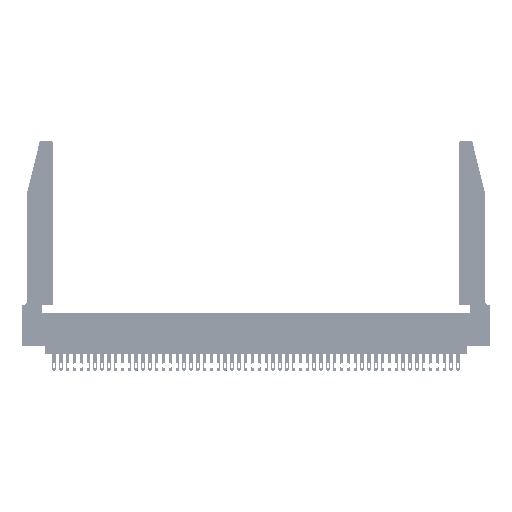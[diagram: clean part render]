
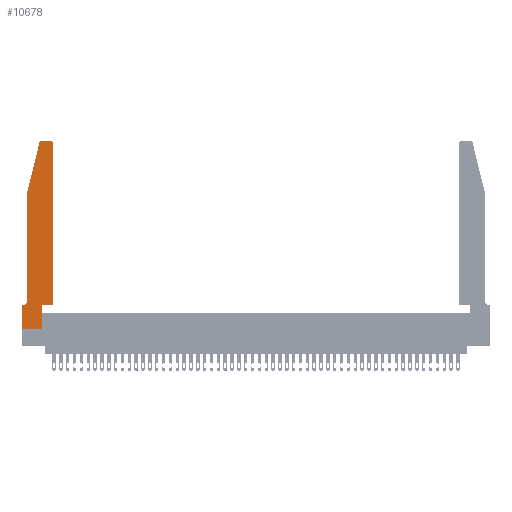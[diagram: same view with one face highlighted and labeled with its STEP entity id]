
A CAD part, top view. The second image highlights one B-rep face of the part: STEP entity #10678.
In plain terms, the highlighted planar face has unit normal (0, 0, 1).
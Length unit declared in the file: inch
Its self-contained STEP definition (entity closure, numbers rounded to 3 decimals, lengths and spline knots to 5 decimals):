
#376 = CARTESIAN_POINT ( 'NONE',  ( 0., 0., 0.37 ) ) ;
#526 = EDGE_CURVE ( 'NONE', #38682, #22160, #24939, .T. ) ;
#804 = EDGE_CURVE ( 'NONE', #26016, #16310, #4045, .T. ) ;
#1109 = CARTESIAN_POINT ( 'NONE',  ( 0.2865, 0.35, 0.37 ) ) ;
#1453 = DIRECTION ( 'NONE',  ( 0., 1., 0. ) ) ;
#1517 = CARTESIAN_POINT ( 'NONE',  ( 0.0055, 0.35, 0.37 ) ) ;
#1753 = CARTESIAN_POINT ( 'NONE',  ( 0.284, 2.72, 0.37 ) ) ;
#2973 = CARTESIAN_POINT ( 'NONE',  ( 0.284, 2.75, 0.37 ) ) ;
#3217 = DIRECTION ( 'NONE',  ( 0., -1., 0. ) ) ;
#3807 = CARTESIAN_POINT ( 'NONE',  ( 0.4505, 2.72, 0.37 ) ) ;
#4045 = LINE ( 'NONE', #29540, #39328 ) ;
#4245 = ORIENTED_EDGE ( 'NONE', *, *, #41643, .T. ) ;
#4680 = AXIS2_PLACEMENT_3D ( 'NONE', #41385, #18926, #25954 ) ;
#5429 = DIRECTION ( 'NONE',  ( 1., 0., 0. ) ) ;
#6351 = ORIENTED_EDGE ( 'NONE', *, *, #45838, .T. ) ;
#6752 = VERTEX_POINT ( 'NONE', #3807 ) ;
#7776 = VERTEX_POINT ( 'NONE', #26711 ) ;
#8085 = VERTEX_POINT ( 'NONE', #24197 ) ;
#8379 = LINE ( 'NONE', #11091, #11355 ) ;
#8451 = EDGE_CURVE ( 'NONE', #6752, #7776, #31970, .T. ) ;
#9571 = CARTESIAN_POINT ( 'NONE',  ( 0., 0., 0.37 ) ) ;
#9941 = CARTESIAN_POINT ( 'NONE',  ( 0.4505, 0.35, 0.37 ) ) ;
#10329 = ORIENTED_EDGE ( 'NONE', *, *, #526, .T. ) ;
#10678 = ADVANCED_FACE ( 'NONE', ( #11973 ), #41891, .T. ) ;
#10757 = DIRECTION ( 'NONE',  ( -0.239, -0.971, 0. ) ) ;
#11017 = CARTESIAN_POINT ( 'NONE',  ( 0.0755, 2., 0.37 ) ) ;
#11091 = CARTESIAN_POINT ( 'NONE',  ( 0.0755, 2., 0.37 ) ) ;
#11102 = AXIS2_PLACEMENT_3D ( 'NONE', #1753, #39840, #5429 ) ;
#11355 = VECTOR ( 'NONE', #10757, 39.37008 ) ;
#11973 = FACE_OUTER_BOUND ( 'NONE', #23315, .T. ) ;
#12323 = DIRECTION ( 'NONE',  ( 0., 0., 1. ) ) ;
#14191 = EDGE_CURVE ( 'NONE', #43947, #6752, #27194, .T. ) ;
#14312 = EDGE_CURVE ( 'NONE', #21810, #43947, #43929, .T. ) ;
#15010 = ORIENTED_EDGE ( 'NONE', *, *, #14312, .T. ) ;
#15188 = VECTOR ( 'NONE', #1453, 39.37008 ) ;
#15980 = CARTESIAN_POINT ( 'NONE',  ( 0., 0.35, 0.37 ) ) ;
#16310 = VERTEX_POINT ( 'NONE', #9571 ) ;
#17216 = DIRECTION ( 'NONE',  ( -1., 0., 0. ) ) ;
#17727 = LINE ( 'NONE', #376, #42270 ) ;
#17859 = ORIENTED_EDGE ( 'NONE', *, *, #39310, .T. ) ;
#17918 = EDGE_CURVE ( 'NONE', #16310, #39950, #17727, .T. ) ;
#18926 = DIRECTION ( 'NONE',  ( 0., 0., 1. ) ) ;
#20423 = LINE ( 'NONE', #30403, #29424 ) ;
#20490 = ORIENTED_EDGE ( 'NONE', *, *, #35469, .T. ) ;
#21145 = DIRECTION ( 'NONE',  ( 1., 0., 0. ) ) ;
#21810 = VERTEX_POINT ( 'NONE', #34072 ) ;
#22160 = VERTEX_POINT ( 'NONE', #37722 ) ;
#23059 = LINE ( 'NONE', #48039, #33833 ) ;
#23069 = DIRECTION ( 'NONE',  ( 1., 0., 0. ) ) ;
#23315 = EDGE_LOOP ( 'NONE', ( #28605, #10329, #17859, #20490, #34963, #4245, #41265, #25785, #6351, #15010, #24087, #34258 ) ) ;
#24087 = ORIENTED_EDGE ( 'NONE', *, *, #14191, .T. ) ;
#24197 = CARTESIAN_POINT ( 'NONE',  ( 0.0755, 2., 0.37 ) ) ;
#24939 = CIRCLE ( 'NONE', #11102, 0.03 ) ;
#25058 = AXIS2_PLACEMENT_3D ( 'NONE', #39746, #12323, #43581 ) ;
#25785 = ORIENTED_EDGE ( 'NONE', *, *, #17918, .T. ) ;
#25794 = DIRECTION ( 'NONE',  ( -1., 0., 0. ) ) ;
#25954 = DIRECTION ( 'NONE',  ( 1., 0., 0. ) ) ;
#26016 = VERTEX_POINT ( 'NONE', #15980 ) ;
#26235 = DIRECTION ( 'NONE',  ( -1., 0., 0. ) ) ;
#26711 = CARTESIAN_POINT ( 'NONE',  ( 0.4205, 2.75, 0.37 ) ) ;
#27194 = LINE ( 'NONE', #35518, #33777 ) ;
#27537 = VERTEX_POINT ( 'NONE', #39351 ) ;
#28605 = ORIENTED_EDGE ( 'NONE', *, *, #37668, .T. ) ;
#29074 = EDGE_CURVE ( 'NONE', #27537, #40190, #44152, .T. ) ;
#29424 = VECTOR ( 'NONE', #26235, 39.37008 ) ;
#29540 = CARTESIAN_POINT ( 'NONE',  ( 0., 0., 0.37 ) ) ;
#29863 = CARTESIAN_POINT ( 'NONE',  ( 0.2865, 0., 0.37 ) ) ;
#30403 = CARTESIAN_POINT ( 'NONE',  ( 0.2605, 2.75, 0.37 ) ) ;
#31970 = CIRCLE ( 'NONE', #25058, 0.03 ) ;
#33727 = VECTOR ( 'NONE', #21145, 39.37008 ) ;
#33777 = VECTOR ( 'NONE', #39398, 39.37008 ) ;
#33833 = VECTOR ( 'NONE', #17216, 39.37008 ) ;
#34072 = CARTESIAN_POINT ( 'NONE',  ( 0.2865, 0.35, 0.37 ) ) ;
#34258 = ORIENTED_EDGE ( 'NONE', *, *, #8451, .T. ) ;
#34963 = ORIENTED_EDGE ( 'NONE', *, *, #29074, .T. ) ;
#35469 = EDGE_CURVE ( 'NONE', #8085, #27537, #48845, .T. ) ;
#35518 = CARTESIAN_POINT ( 'NONE',  ( 0.4505, 0.35, 0.37 ) ) ;
#37668 = EDGE_CURVE ( 'NONE', #7776, #38682, #20423, .T. ) ;
#37722 = CARTESIAN_POINT ( 'NONE',  ( 0.25487, 2.72718, 0.37 ) ) ;
#38066 = AXIS2_PLACEMENT_3D ( 'NONE', #45384, #45558, #25794 ) ;
#38507 = LINE ( 'NONE', #1109, #15188 ) ;
#38682 = VERTEX_POINT ( 'NONE', #2973 ) ;
#39310 = EDGE_CURVE ( 'NONE', #22160, #8085, #8379, .T. ) ;
#39328 = VECTOR ( 'NONE', #3217, 39.37008 ) ;
#39351 = CARTESIAN_POINT ( 'NONE',  ( 0.0755, 0.42, 0.37 ) ) ;
#39398 = DIRECTION ( 'NONE',  ( 0., 1., 0. ) ) ;
#39746 = CARTESIAN_POINT ( 'NONE',  ( 0.4205, 2.72, 0.37 ) ) ;
#39840 = DIRECTION ( 'NONE',  ( 0., 0., 1. ) ) ;
#39950 = VERTEX_POINT ( 'NONE', #29863 ) ;
#40190 = VERTEX_POINT ( 'NONE', #1517 ) ;
#41265 = ORIENTED_EDGE ( 'NONE', *, *, #804, .T. ) ;
#41385 = CARTESIAN_POINT ( 'NONE',  ( 0., 0.35, 0.37 ) ) ;
#41619 = DIRECTION ( 'NONE',  ( 0., -1., 0. ) ) ;
#41643 = EDGE_CURVE ( 'NONE', #40190, #26016, #23059, .T. ) ;
#41891 = PLANE ( 'NONE',  #4680 ) ;
#42270 = VECTOR ( 'NONE', #23069, 39.37008 ) ;
#42848 = VECTOR ( 'NONE', #41619, 39.37008 ) ;
#43581 = DIRECTION ( 'NONE',  ( 1., 0., 0. ) ) ;
#43929 = LINE ( 'NONE', #47926, #33727 ) ;
#43947 = VERTEX_POINT ( 'NONE', #9941 ) ;
#44152 = CIRCLE ( 'NONE', #38066, 0.07 ) ;
#45384 = CARTESIAN_POINT ( 'NONE',  ( 0.0055, 0.42, 0.37 ) ) ;
#45558 = DIRECTION ( 'NONE',  ( 0., 0., -1. ) ) ;
#45838 = EDGE_CURVE ( 'NONE', #39950, #21810, #38507, .T. ) ;
#47926 = CARTESIAN_POINT ( 'NONE',  ( 0.4505, 0.35, 0.37 ) ) ;
#48039 = CARTESIAN_POINT ( 'NONE',  ( 0.0755, 0.35, 0.37 ) ) ;
#48845 = LINE ( 'NONE', #11017, #42848 ) ;
